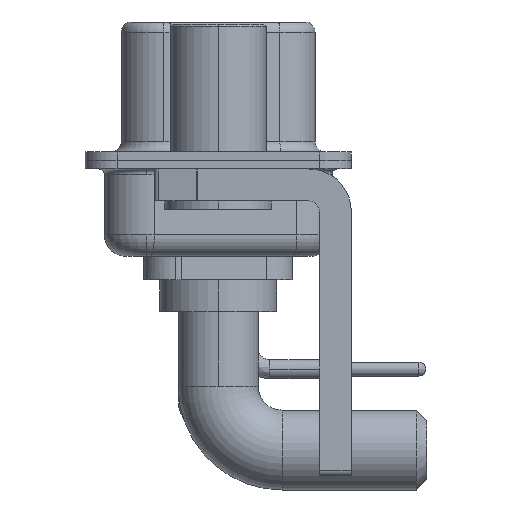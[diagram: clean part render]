
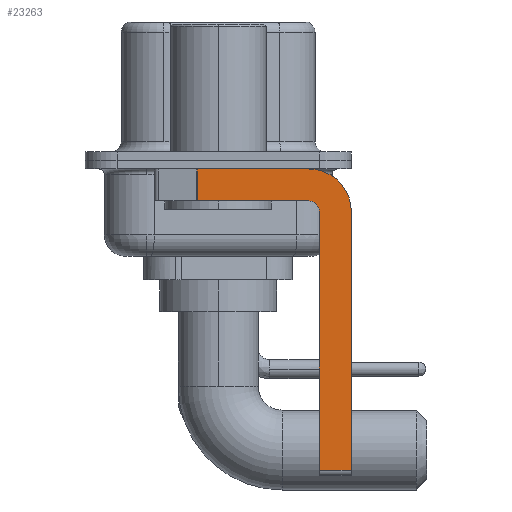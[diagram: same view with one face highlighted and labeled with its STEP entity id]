
A CAD part, left-side view. The second image highlights one B-rep face of the part: STEP entity #23263.
In plain terms, the highlighted planar face has unit normal (-1, 0, 0).
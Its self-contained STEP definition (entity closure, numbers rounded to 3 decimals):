
#133 = VERTEX_POINT ( 'NONE', #20076 ) ;
#256 = CARTESIAN_POINT ( 'NONE',  ( -2.9, -6.25, -2.4 ) ) ;
#572 = EDGE_LOOP ( 'NONE', ( #6918, #4388, #11233, #2660, #1543, #15212, #18968, #21572 ) ) ;
#803 = DIRECTION ( 'NONE',  ( 0., 1., 0. ) ) ;
#881 = CARTESIAN_POINT ( 'NONE',  ( -2.9, -4.25, -2.4 ) ) ;
#1543 = ORIENTED_EDGE ( 'NONE', *, *, #19393, .F. ) ;
#1589 = LINE ( 'NONE', #3369, #22093 ) ;
#2660 = ORIENTED_EDGE ( 'NONE', *, *, #12987, .F. ) ;
#2809 = DIRECTION ( 'NONE',  ( 1., 0., 0. ) ) ;
#3239 = EDGE_CURVE ( 'NONE', #23915, #18808, #1589, .T. ) ;
#3369 = CARTESIAN_POINT ( 'NONE',  ( -2.9, 0.978, -1.9 ) ) ;
#3549 = DIRECTION ( 'NONE',  ( 0., 0., 1. ) ) ;
#3596 = VECTOR ( 'NONE', #25283, 1000. ) ;
#3969 = AXIS2_PLACEMENT_3D ( 'NONE', #881, #2809, #15214 ) ;
#4388 = ORIENTED_EDGE ( 'NONE', *, *, #3239, .T. ) ;
#4708 = FACE_OUTER_BOUND ( 'NONE', #572, .T. ) ;
#6899 = LINE ( 'NONE', #15464, #22607 ) ;
#6918 = ORIENTED_EDGE ( 'NONE', *, *, #25432, .F. ) ;
#7196 = CARTESIAN_POINT ( 'NONE',  ( -2.9, 3., -0.4 ) ) ;
#7208 = CARTESIAN_POINT ( 'NONE',  ( -2.9, -4.25, -2.4 ) ) ;
#8658 = CARTESIAN_POINT ( 'NONE',  ( -2.9, -6.25, -14.55 ) ) ;
#9077 = EDGE_CURVE ( 'NONE', #9584, #26318, #6899, .T. ) ;
#9265 = LINE ( 'NONE', #7196, #14964 ) ;
#9367 = CARTESIAN_POINT ( 'NONE',  ( -2.9, -4.25, -2.4 ) ) ;
#9394 = DIRECTION ( 'NONE',  ( 0., -1., 0. ) ) ;
#9584 = VERTEX_POINT ( 'NONE', #256 ) ;
#9915 = CIRCLE ( 'NONE', #25346, 0.5 ) ;
#10064 = VERTEX_POINT ( 'NONE', #15239 ) ;
#10370 = CARTESIAN_POINT ( 'NONE',  ( -2.9, -4.25, -1.9 ) ) ;
#10396 = VERTEX_POINT ( 'NONE', #10370 ) ;
#10931 = DIRECTION ( 'NONE',  ( 0., 0., 1. ) ) ;
#11233 = ORIENTED_EDGE ( 'NONE', *, *, #17956, .F. ) ;
#12875 = DIRECTION ( 'NONE',  ( -1., 0., 0. ) ) ;
#12987 = EDGE_CURVE ( 'NONE', #133, #10396, #9915, .T. ) ;
#13600 = LINE ( 'NONE', #24349, #26021 ) ;
#13751 = CARTESIAN_POINT ( 'NONE',  ( -2.9, 0.978, -0.4 ) ) ;
#14964 = VECTOR ( 'NONE', #9394, 1000. ) ;
#15190 = DIRECTION ( 'NONE',  ( 1., 0., 0. ) ) ;
#15212 = ORIENTED_EDGE ( 'NONE', *, *, #20102, .T. ) ;
#15214 = DIRECTION ( 'NONE',  ( 0., 0., -1. ) ) ;
#15239 = CARTESIAN_POINT ( 'NONE',  ( -2.9, -4.25, -0.4 ) ) ;
#15464 = CARTESIAN_POINT ( 'NONE',  ( -2.9, -6.25, -2.4 ) ) ;
#15677 = LINE ( 'NONE', #23943, #21967 ) ;
#17389 = DIRECTION ( 'NONE',  ( 0., 0., -1. ) ) ;
#17956 = EDGE_CURVE ( 'NONE', #10396, #18808, #15677, .T. ) ;
#18386 = CARTESIAN_POINT ( 'NONE',  ( -2.9, -4.25, -14.55 ) ) ;
#18444 = AXIS2_PLACEMENT_3D ( 'NONE', #9367, #15190, #17389 ) ;
#18808 = VERTEX_POINT ( 'NONE', #19074 ) ;
#18968 = ORIENTED_EDGE ( 'NONE', *, *, #9077, .F. ) ;
#19074 = CARTESIAN_POINT ( 'NONE',  ( -2.9, 0.978, -1.9 ) ) ;
#19393 = EDGE_CURVE ( 'NONE', #26062, #133, #13600, .T. ) ;
#20076 = CARTESIAN_POINT ( 'NONE',  ( -2.9, -4.75, -2.4 ) ) ;
#20102 = EDGE_CURVE ( 'NONE', #26062, #26318, #22532, .T. ) ;
#20113 = CARTESIAN_POINT ( 'NONE',  ( -2.9, -4.75, -14.55 ) ) ;
#21572 = ORIENTED_EDGE ( 'NONE', *, *, #25406, .F. ) ;
#21789 = DIRECTION ( 'NONE',  ( 0., 0., -1. ) ) ;
#21967 = VECTOR ( 'NONE', #803, 1000. ) ;
#21983 = DIRECTION ( 'NONE',  ( 0., 0., -1. ) ) ;
#22093 = VECTOR ( 'NONE', #21983, 1000. ) ;
#22532 = LINE ( 'NONE', #18386, #3596 ) ;
#22607 = VECTOR ( 'NONE', #21789, 1000. ) ;
#23263 = ADVANCED_FACE ( 'NONE', ( #4708 ), #26203, .F. ) ;
#23915 = VERTEX_POINT ( 'NONE', #13751 ) ;
#23943 = CARTESIAN_POINT ( 'NONE',  ( -2.9, -4.25, -1.9 ) ) ;
#24202 = CIRCLE ( 'NONE', #3969, 2. ) ;
#24349 = CARTESIAN_POINT ( 'NONE',  ( -2.9, -4.75, -14.8 ) ) ;
#25283 = DIRECTION ( 'NONE',  ( 0., -1., 0. ) ) ;
#25346 = AXIS2_PLACEMENT_3D ( 'NONE', #7208, #12875, #10931 ) ;
#25406 = EDGE_CURVE ( 'NONE', #10064, #9584, #24202, .T. ) ;
#25432 = EDGE_CURVE ( 'NONE', #23915, #10064, #9265, .T. ) ;
#26021 = VECTOR ( 'NONE', #3549, 1000. ) ;
#26062 = VERTEX_POINT ( 'NONE', #20113 ) ;
#26203 = PLANE ( 'NONE',  #18444 ) ;
#26318 = VERTEX_POINT ( 'NONE', #8658 ) ;
